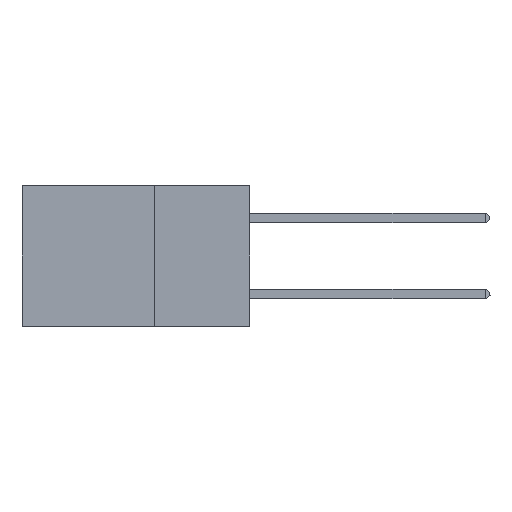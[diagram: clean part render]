
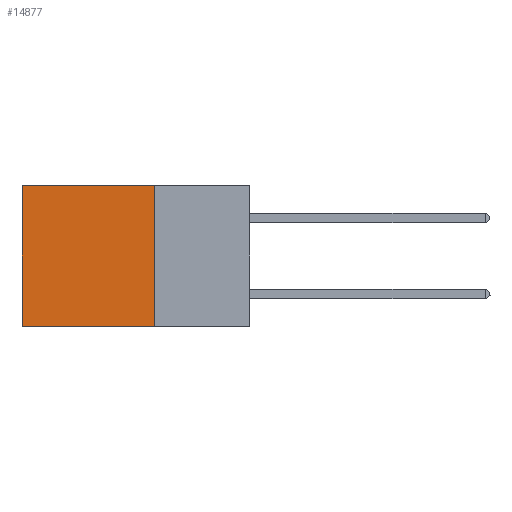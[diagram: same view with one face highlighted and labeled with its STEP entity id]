
A CAD part, left-side view. The second image highlights one B-rep face of the part: STEP entity #14877.
In plain terms, the highlighted planar face has unit normal (-1, 0, 0).
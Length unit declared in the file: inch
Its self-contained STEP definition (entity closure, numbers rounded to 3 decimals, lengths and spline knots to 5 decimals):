
#250 = VECTOR ( 'NONE', #4010, 39.37008 ) ;
#702 = VERTEX_POINT ( 'NONE', #15183 ) ;
#728 = CARTESIAN_POINT ( 'NONE',  ( 0.2875, 0.25, 0. ) ) ;
#1705 = ORIENTED_EDGE ( 'NONE', *, *, #3064, .T. ) ;
#2662 = AXIS2_PLACEMENT_3D ( 'NONE', #14686, #10102, #2939 ) ;
#2939 = DIRECTION ( 'NONE',  ( 0., 0., -1. ) ) ;
#3064 = EDGE_CURVE ( 'NONE', #13933, #702, #5190, .T. ) ;
#3148 = EDGE_LOOP ( 'NONE', ( #14690, #3792, #6086, #1705 ) ) ;
#3377 = DIRECTION ( 'NONE',  ( 0., 1., 0. ) ) ;
#3689 = CARTESIAN_POINT ( 'NONE',  ( 0.2875, 0.6, -0.37 ) ) ;
#3792 = ORIENTED_EDGE ( 'NONE', *, *, #6998, .F. ) ;
#3953 = CARTESIAN_POINT ( 'NONE',  ( 0.2875, 0.25, -0.37 ) ) ;
#4010 = DIRECTION ( 'NONE',  ( 0., 0., -1. ) ) ;
#5040 = LINE ( 'NONE', #728, #10947 ) ;
#5190 = LINE ( 'NONE', #10644, #12176 ) ;
#5945 = CARTESIAN_POINT ( 'NONE',  ( 0.2875, 0.25, 0. ) ) ;
#6086 = ORIENTED_EDGE ( 'NONE', *, *, #9066, .F. ) ;
#6998 = EDGE_CURVE ( 'NONE', #8288, #14005, #8442, .T. ) ;
#8139 = FACE_OUTER_BOUND ( 'NONE', #3148, .T. ) ;
#8288 = VERTEX_POINT ( 'NONE', #3953 ) ;
#8296 = DIRECTION ( 'NONE',  ( 0., 1., 0. ) ) ;
#8442 = LINE ( 'NONE', #12843, #11187 ) ;
#9066 = EDGE_CURVE ( 'NONE', #13933, #8288, #5040, .T. ) ;
#10055 = PLANE ( 'NONE',  #2662 ) ;
#10102 = DIRECTION ( 'NONE',  ( 1., 0., 0. ) ) ;
#10644 = CARTESIAN_POINT ( 'NONE',  ( 0.2875, 0.25, 0. ) ) ;
#10947 = VECTOR ( 'NONE', #12587, 39.37008 ) ;
#11096 = CARTESIAN_POINT ( 'NONE',  ( 0.2875, 0.6, 0. ) ) ;
#11187 = VECTOR ( 'NONE', #3377, 39.37008 ) ;
#12176 = VECTOR ( 'NONE', #8296, 39.37008 ) ;
#12534 = LINE ( 'NONE', #11096, #250 ) ;
#12587 = DIRECTION ( 'NONE',  ( 0., 0., -1. ) ) ;
#12843 = CARTESIAN_POINT ( 'NONE',  ( 0.2875, 0.25, -0.37 ) ) ;
#13933 = VERTEX_POINT ( 'NONE', #5945 ) ;
#14005 = VERTEX_POINT ( 'NONE', #3689 ) ;
#14142 = EDGE_CURVE ( 'NONE', #702, #14005, #12534, .T. ) ;
#14686 = CARTESIAN_POINT ( 'NONE',  ( 0.2875, 0.25, 0. ) ) ;
#14690 = ORIENTED_EDGE ( 'NONE', *, *, #14142, .T. ) ;
#14877 = ADVANCED_FACE ( 'NONE', ( #8139 ), #10055, .F. ) ;
#15183 = CARTESIAN_POINT ( 'NONE',  ( 0.2875, 0.6, 0. ) ) ;
